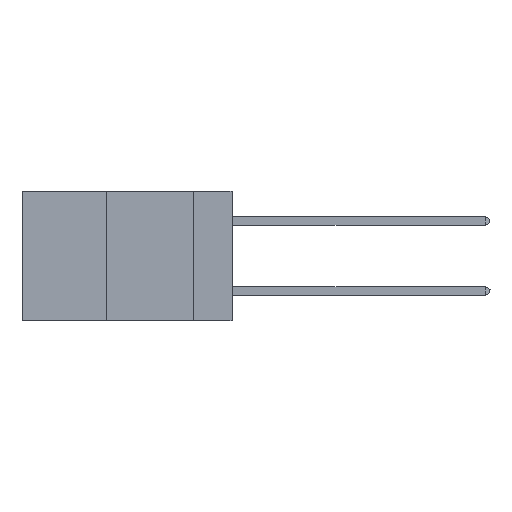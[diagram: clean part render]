
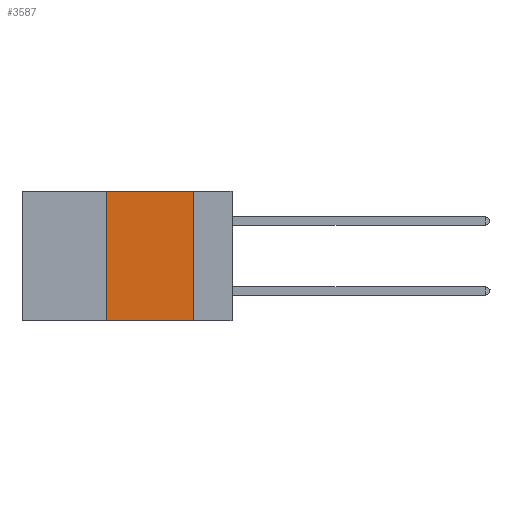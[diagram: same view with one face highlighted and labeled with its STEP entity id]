
A CAD part, left-side view. The second image highlights one B-rep face of the part: STEP entity #3587.
In plain terms, the highlighted planar face has unit normal (-1, 0, 0).
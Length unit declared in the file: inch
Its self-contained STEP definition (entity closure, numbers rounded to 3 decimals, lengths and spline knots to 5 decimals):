
#391 = VECTOR ( 'NONE', #8934, 39.37008 ) ;
#532 = CARTESIAN_POINT ( 'NONE',  ( 0., 0.36, 0. ) ) ;
#738 = DIRECTION ( 'NONE',  ( 0., -1., 0. ) ) ;
#1507 = PLANE ( 'NONE',  #9856 ) ;
#1929 = FACE_OUTER_BOUND ( 'NONE', #10416, .T. ) ;
#2710 = VERTEX_POINT ( 'NONE', #12350 ) ;
#3429 = VERTEX_POINT ( 'NONE', #13954 ) ;
#3587 = ADVANCED_FACE ( 'NONE', ( #1929 ), #1507, .F. ) ;
#3682 = LINE ( 'NONE', #532, #4463 ) ;
#3709 = LINE ( 'NONE', #12621, #391 ) ;
#4187 = VERTEX_POINT ( 'NONE', #5586 ) ;
#4463 = VECTOR ( 'NONE', #15108, 39.37008 ) ;
#5165 = VECTOR ( 'NONE', #13084, 39.37008 ) ;
#5329 = VECTOR ( 'NONE', #738, 39.37008 ) ;
#5548 = DIRECTION ( 'NONE',  ( 0., 0., -1. ) ) ;
#5586 = CARTESIAN_POINT ( 'NONE',  ( 0., 0.36, -0.37 ) ) ;
#6195 = EDGE_CURVE ( 'NONE', #2710, #10592, #13063, .T. ) ;
#8579 = LINE ( 'NONE', #10721, #5329 ) ;
#8934 = DIRECTION ( 'NONE',  ( 0., -1., 0. ) ) ;
#9300 = EDGE_CURVE ( 'NONE', #4187, #3429, #3682, .T. ) ;
#9856 = AXIS2_PLACEMENT_3D ( 'NONE', #14137, #10346, #5548 ) ;
#10346 = DIRECTION ( 'NONE',  ( 1., 0., 0. ) ) ;
#10416 = EDGE_LOOP ( 'NONE', ( #10475, #10632, #12335, #12456 ) ) ;
#10475 = ORIENTED_EDGE ( 'NONE', *, *, #6195, .F. ) ;
#10592 = VERTEX_POINT ( 'NONE', #11893 ) ;
#10632 = ORIENTED_EDGE ( 'NONE', *, *, #11594, .F. ) ;
#10721 = CARTESIAN_POINT ( 'NONE',  ( 0., 0.6, 0. ) ) ;
#11594 = EDGE_CURVE ( 'NONE', #3429, #2710, #8579, .T. ) ;
#11893 = CARTESIAN_POINT ( 'NONE',  ( 0., 0.11, -0.37 ) ) ;
#12335 = ORIENTED_EDGE ( 'NONE', *, *, #9300, .F. ) ;
#12350 = CARTESIAN_POINT ( 'NONE',  ( 0., 0.11, 0. ) ) ;
#12456 = ORIENTED_EDGE ( 'NONE', *, *, #14467, .T. ) ;
#12621 = CARTESIAN_POINT ( 'NONE',  ( 0., 0.6, -0.37 ) ) ;
#13063 = LINE ( 'NONE', #13246, #5165 ) ;
#13084 = DIRECTION ( 'NONE',  ( 0., 0., -1. ) ) ;
#13246 = CARTESIAN_POINT ( 'NONE',  ( 0., 0.11, 0. ) ) ;
#13954 = CARTESIAN_POINT ( 'NONE',  ( 0., 0.36, 0. ) ) ;
#14137 = CARTESIAN_POINT ( 'NONE',  ( 0., 0.6, 0. ) ) ;
#14467 = EDGE_CURVE ( 'NONE', #4187, #10592, #3709, .T. ) ;
#15108 = DIRECTION ( 'NONE',  ( 0., 0., 1. ) ) ;
